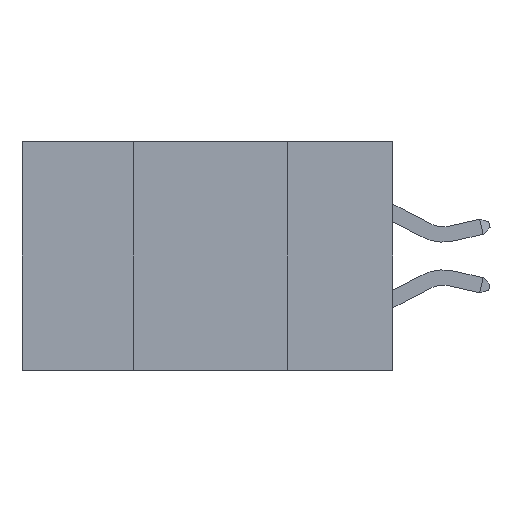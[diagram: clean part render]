
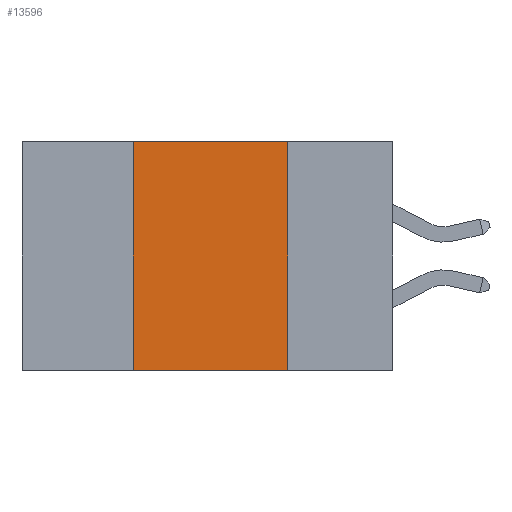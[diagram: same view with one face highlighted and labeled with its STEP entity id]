
A CAD part, left-side view. The second image highlights one B-rep face of the part: STEP entity #13596.
In plain terms, the highlighted planar face has unit normal (-1, 0, 0).
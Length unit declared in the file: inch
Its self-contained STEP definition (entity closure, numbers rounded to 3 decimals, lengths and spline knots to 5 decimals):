
#46 = ORIENTED_EDGE ( 'NONE', *, *, #8731, .F. ) ;
#165 = VECTOR ( 'NONE', #8087, 39.37008 ) ;
#394 = DIRECTION ( 'NONE',  ( 0., -1., 0. ) ) ;
#578 = LINE ( 'NONE', #6844, #165 ) ;
#2311 = VECTOR ( 'NONE', #8302, 39.37008 ) ;
#3363 = FACE_OUTER_BOUND ( 'NONE', #4094, .T. ) ;
#3962 = CARTESIAN_POINT ( 'NONE',  ( 0., 0.42, 0. ) ) ;
#4094 = EDGE_LOOP ( 'NONE', ( #9400, #46, #10558, #15363 ) ) ;
#4376 = EDGE_CURVE ( 'NONE', #15091, #10603, #9516, .T. ) ;
#5664 = LINE ( 'NONE', #13773, #14848 ) ;
#6844 = CARTESIAN_POINT ( 'NONE',  ( 0., 0.6, -0.37 ) ) ;
#6882 = DIRECTION ( 'NONE',  ( 1., 0., 0. ) ) ;
#7170 = VERTEX_POINT ( 'NONE', #3962 ) ;
#7379 = CARTESIAN_POINT ( 'NONE',  ( 0., 0.17, 0. ) ) ;
#7830 = CARTESIAN_POINT ( 'NONE',  ( 0., 0.6, 0. ) ) ;
#7847 = LINE ( 'NONE', #7830, #10720 ) ;
#7981 = CARTESIAN_POINT ( 'NONE',  ( 0., 0.17, -0.37 ) ) ;
#8087 = DIRECTION ( 'NONE',  ( 0., -1., 0. ) ) ;
#8302 = DIRECTION ( 'NONE',  ( 0., 0., -1. ) ) ;
#8439 = CARTESIAN_POINT ( 'NONE',  ( 0., 0.17, 0. ) ) ;
#8731 = EDGE_CURVE ( 'NONE', #7170, #15091, #7847, .T. ) ;
#9400 = ORIENTED_EDGE ( 'NONE', *, *, #4376, .F. ) ;
#9516 = LINE ( 'NONE', #8439, #2311 ) ;
#10351 = CARTESIAN_POINT ( 'NONE',  ( 0., 0.42, -0.37 ) ) ;
#10534 = PLANE ( 'NONE',  #11989 ) ;
#10558 = ORIENTED_EDGE ( 'NONE', *, *, #13403, .F. ) ;
#10603 = VERTEX_POINT ( 'NONE', #7981 ) ;
#10720 = VECTOR ( 'NONE', #394, 39.37008 ) ;
#11989 = AXIS2_PLACEMENT_3D ( 'NONE', #14114, #6882, #15271 ) ;
#12104 = VERTEX_POINT ( 'NONE', #10351 ) ;
#12861 = EDGE_CURVE ( 'NONE', #12104, #10603, #578, .T. ) ;
#13403 = EDGE_CURVE ( 'NONE', #12104, #7170, #5664, .T. ) ;
#13596 = ADVANCED_FACE ( 'NONE', ( #3363 ), #10534, .F. ) ;
#13773 = CARTESIAN_POINT ( 'NONE',  ( 0., 0.42, 0. ) ) ;
#14114 = CARTESIAN_POINT ( 'NONE',  ( 0., 0.6, 0. ) ) ;
#14848 = VECTOR ( 'NONE', #14917, 39.37008 ) ;
#14917 = DIRECTION ( 'NONE',  ( 0., 0., 1. ) ) ;
#15091 = VERTEX_POINT ( 'NONE', #7379 ) ;
#15271 = DIRECTION ( 'NONE',  ( 0., 0., -1. ) ) ;
#15363 = ORIENTED_EDGE ( 'NONE', *, *, #12861, .T. ) ;
